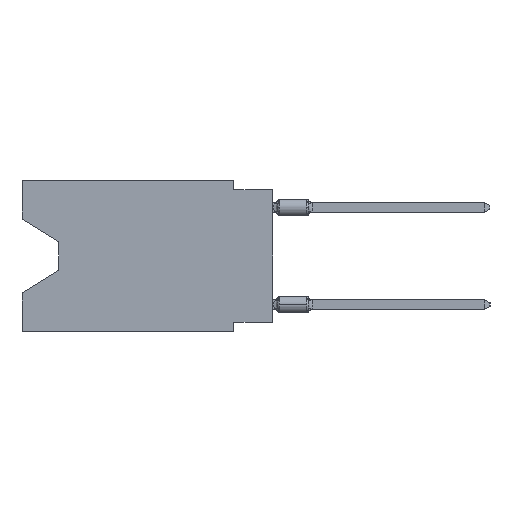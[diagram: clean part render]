
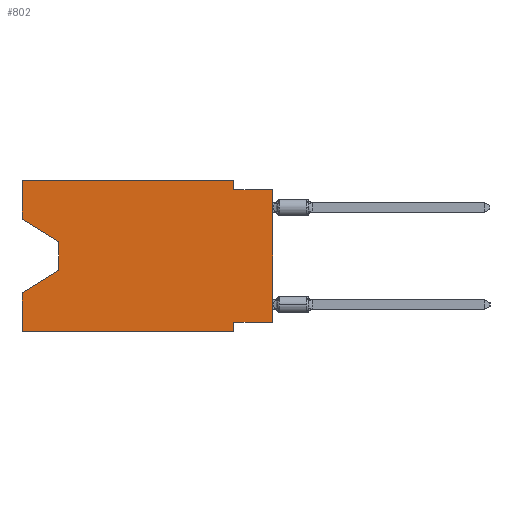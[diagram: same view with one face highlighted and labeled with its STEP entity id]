
A CAD part, left-side view. The second image highlights one B-rep face of the part: STEP entity #802.
In plain terms, the highlighted planar face has unit normal (-1, 0, 0).
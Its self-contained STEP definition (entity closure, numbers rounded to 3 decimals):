
#43 = EDGE_CURVE ( 'NONE', #23384, #20277, #305, .T. ) ;
#305 = LINE ( 'NONE', #27357, #21355 ) ;
#802 = ADVANCED_FACE ( 'NONE', ( #4151 ), #14222, .F. ) ;
#1087 = CARTESIAN_POINT ( 'NONE',  ( 0., 0., 0. ) ) ;
#1597 = VECTOR ( 'NONE', #29161, 1000. ) ;
#2152 = CARTESIAN_POINT ( 'NONE',  ( 0., 0., -9.271 ) ) ;
#2169 = VERTEX_POINT ( 'NONE', #25751 ) ;
#2700 = CARTESIAN_POINT ( 'NONE',  ( 0., 16.383, 0. ) ) ;
#2741 = LINE ( 'NONE', #32434, #15651 ) ;
#2919 = ORIENTED_EDGE ( 'NONE', *, *, #3129, .T. ) ;
#3129 = EDGE_CURVE ( 'NONE', #12724, #6793, #19356, .T. ) ;
#3281 = VECTOR ( 'NONE', #18871, 1000. ) ;
#3287 = LINE ( 'NONE', #5435, #11254 ) ;
#3308 = VECTOR ( 'NONE', #7264, 1000. ) ;
#3496 = CARTESIAN_POINT ( 'NONE',  ( 0., 16.383, -2.546 ) ) ;
#3830 = DIRECTION ( 'NONE',  ( 0., -1., 0. ) ) ;
#4151 = FACE_OUTER_BOUND ( 'NONE', #28544, .T. ) ;
#4471 = CARTESIAN_POINT ( 'NONE',  ( 0., 16.383, 0. ) ) ;
#5012 = EDGE_CURVE ( 'NONE', #22490, #9784, #3287, .T. ) ;
#5329 = EDGE_CURVE ( 'NONE', #6793, #18944, #24699, .T. ) ;
#5435 = CARTESIAN_POINT ( 'NONE',  ( 0., 16.383, 0. ) ) ;
#5537 = DIRECTION ( 'NONE',  ( 0., 0., -1. ) ) ;
#5674 = VERTEX_POINT ( 'NONE', #12139 ) ;
#6204 = EDGE_CURVE ( 'NONE', #12724, #28472, #12435, .T. ) ;
#6736 = CARTESIAN_POINT ( 'NONE',  ( 0., 13.97, -5.893 ) ) ;
#6793 = VERTEX_POINT ( 'NONE', #30836 ) ;
#7132 = ORIENTED_EDGE ( 'NONE', *, *, #5329, .T. ) ;
#7163 = CARTESIAN_POINT ( 'NONE',  ( 0., 16.383, -7.36 ) ) ;
#7264 = DIRECTION ( 'NONE',  ( 0., 1., 0. ) ) ;
#8810 = VERTEX_POINT ( 'NONE', #19501 ) ;
#8877 = LINE ( 'NONE', #6736, #24885 ) ;
#9784 = VERTEX_POINT ( 'NONE', #7163 ) ;
#9875 = CARTESIAN_POINT ( 'NONE',  ( 0., 2.54, -9.271 ) ) ;
#10808 = EDGE_CURVE ( 'NONE', #8810, #5674, #10991, .T. ) ;
#10991 = LINE ( 'NONE', #1087, #12754 ) ;
#11143 = DIRECTION ( 'NONE',  ( 0., 0., 1. ) ) ;
#11254 = VECTOR ( 'NONE', #13351, 1000. ) ;
#12139 = CARTESIAN_POINT ( 'NONE',  ( 0., 0., -0.635 ) ) ;
#12435 = LINE ( 'NONE', #2700, #30821 ) ;
#12724 = VERTEX_POINT ( 'NONE', #3496 ) ;
#12754 = VECTOR ( 'NONE', #11143, 1000. ) ;
#13067 = EDGE_CURVE ( 'NONE', #8810, #23384, #29858, .T. ) ;
#13351 = DIRECTION ( 'NONE',  ( 0., 0., 1. ) ) ;
#14222 = PLANE ( 'NONE',  #30327 ) ;
#14629 = ORIENTED_EDGE ( 'NONE', *, *, #10808, .T. ) ;
#15560 = EDGE_CURVE ( 'NONE', #28472, #2169, #19108, .T. ) ;
#15651 = VECTOR ( 'NONE', #5537, 1000. ) ;
#17515 = EDGE_CURVE ( 'NONE', #2169, #29414, #2741, .T. ) ;
#17895 = CARTESIAN_POINT ( 'NONE',  ( 0., 0., -0.635 ) ) ;
#18029 = ORIENTED_EDGE ( 'NONE', *, *, #27355, .T. ) ;
#18213 = EDGE_CURVE ( 'NONE', #22490, #20277, #18861, .T. ) ;
#18861 = LINE ( 'NONE', #27073, #27786 ) ;
#18871 = DIRECTION ( 'NONE',  ( 0., -0.855, -0.519 ) ) ;
#18944 = VERTEX_POINT ( 'NONE', #26307 ) ;
#18957 = DIRECTION ( 'NONE',  ( 0., 0.855, -0.519 ) ) ;
#19031 = ORIENTED_EDGE ( 'NONE', *, *, #18213, .T. ) ;
#19108 = LINE ( 'NONE', #26522, #1597 ) ;
#19356 = LINE ( 'NONE', #21491, #3281 ) ;
#19501 = CARTESIAN_POINT ( 'NONE',  ( 0., 0., -9.271 ) ) ;
#19936 = CARTESIAN_POINT ( 'NONE',  ( 0., 13.97, -4.013 ) ) ;
#20188 = DIRECTION ( 'NONE',  ( 0., 0., 1. ) ) ;
#20277 = VERTEX_POINT ( 'NONE', #23875 ) ;
#20902 = ORIENTED_EDGE ( 'NONE', *, *, #5012, .F. ) ;
#21355 = VECTOR ( 'NONE', #24875, 1000. ) ;
#21491 = CARTESIAN_POINT ( 'NONE',  ( 0., 16.383, -2.546 ) ) ;
#21604 = ORIENTED_EDGE ( 'NONE', *, *, #17515, .F. ) ;
#21647 = ORIENTED_EDGE ( 'NONE', *, *, #6204, .F. ) ;
#22490 = VERTEX_POINT ( 'NONE', #31276 ) ;
#22603 = CARTESIAN_POINT ( 'NONE',  ( 0., 2.54, -0.635 ) ) ;
#23075 = EDGE_CURVE ( 'NONE', #29414, #5674, #27776, .T. ) ;
#23384 = VERTEX_POINT ( 'NONE', #9875 ) ;
#23875 = CARTESIAN_POINT ( 'NONE',  ( 0., 2.54, -9.906 ) ) ;
#24149 = VECTOR ( 'NONE', #24962, 1000. ) ;
#24544 = CARTESIAN_POINT ( 'NONE',  ( 0., 16.383, 0. ) ) ;
#24699 = LINE ( 'NONE', #19936, #26550 ) ;
#24808 = ORIENTED_EDGE ( 'NONE', *, *, #15560, .F. ) ;
#24875 = DIRECTION ( 'NONE',  ( 0., 0., -1. ) ) ;
#24885 = VECTOR ( 'NONE', #18957, 1000. ) ;
#24962 = DIRECTION ( 'NONE',  ( 0., -1., 0. ) ) ;
#25563 = ORIENTED_EDGE ( 'NONE', *, *, #43, .F. ) ;
#25751 = CARTESIAN_POINT ( 'NONE',  ( 0., 2.54, 0. ) ) ;
#26307 = CARTESIAN_POINT ( 'NONE',  ( 0., 13.97, -5.893 ) ) ;
#26352 = ORIENTED_EDGE ( 'NONE', *, *, #13067, .F. ) ;
#26522 = CARTESIAN_POINT ( 'NONE',  ( 0., 16.383, 0. ) ) ;
#26550 = VECTOR ( 'NONE', #32124, 1000. ) ;
#27073 = CARTESIAN_POINT ( 'NONE',  ( 0., 16.383, -9.906 ) ) ;
#27355 = EDGE_CURVE ( 'NONE', #18944, #9784, #8877, .T. ) ;
#27357 = CARTESIAN_POINT ( 'NONE',  ( 0., 2.54, -9.906 ) ) ;
#27407 = DIRECTION ( 'NONE',  ( 1., 0., 0. ) ) ;
#27776 = LINE ( 'NONE', #17895, #24149 ) ;
#27786 = VECTOR ( 'NONE', #3830, 1000. ) ;
#28472 = VERTEX_POINT ( 'NONE', #24544 ) ;
#28544 = EDGE_LOOP ( 'NONE', ( #2919, #7132, #18029, #20902, #19031, #25563, #26352, #14629, #31956, #21604, #24808, #21647 ) ) ;
#29161 = DIRECTION ( 'NONE',  ( 0., -1., 0. ) ) ;
#29414 = VERTEX_POINT ( 'NONE', #22603 ) ;
#29858 = LINE ( 'NONE', #2152, #3308 ) ;
#30327 = AXIS2_PLACEMENT_3D ( 'NONE', #4471, #27407, #32341 ) ;
#30821 = VECTOR ( 'NONE', #20188, 1000. ) ;
#30836 = CARTESIAN_POINT ( 'NONE',  ( 0., 13.97, -4.013 ) ) ;
#31276 = CARTESIAN_POINT ( 'NONE',  ( 0., 16.383, -9.906 ) ) ;
#31956 = ORIENTED_EDGE ( 'NONE', *, *, #23075, .F. ) ;
#32124 = DIRECTION ( 'NONE',  ( 0., 0., -1. ) ) ;
#32341 = DIRECTION ( 'NONE',  ( 0., 0., -1. ) ) ;
#32434 = CARTESIAN_POINT ( 'NONE',  ( 0., 2.54, 0. ) ) ;
